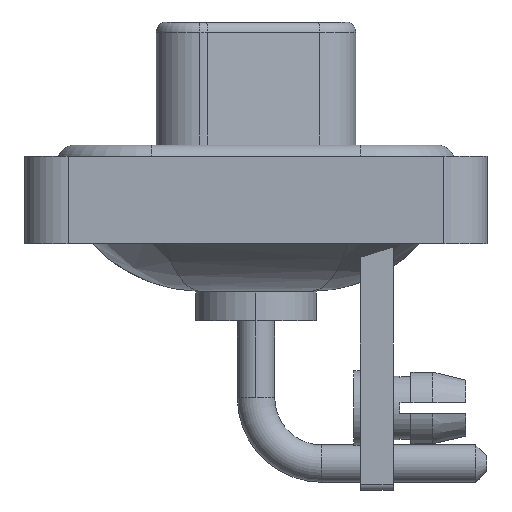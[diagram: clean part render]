
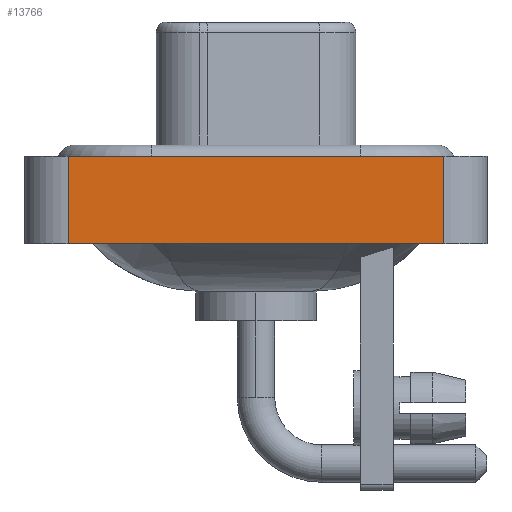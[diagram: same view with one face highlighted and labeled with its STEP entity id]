
A CAD part, left-side view. The second image highlights one B-rep face of the part: STEP entity #13766.
In plain terms, the highlighted planar face has unit normal (-1, 0, 0).
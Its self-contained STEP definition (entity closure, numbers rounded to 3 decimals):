
#1598 = LINE ( 'NONE', #4458, #6937 ) ;
#2211 = VECTOR ( 'NONE', #7094, 1000. ) ;
#2734 = EDGE_CURVE ( 'NONE', #14877, #13758, #1598, .T. ) ;
#2862 = VECTOR ( 'NONE', #9340, 1000. ) ;
#3102 = CARTESIAN_POINT ( 'NONE',  ( -7.25, -8.55, 0.4 ) ) ;
#4458 = CARTESIAN_POINT ( 'NONE',  ( -7.25, -8.55, -3.6 ) ) ;
#4800 = LINE ( 'NONE', #9929, #5241 ) ;
#5241 = VECTOR ( 'NONE', #11504, 1000. ) ;
#5280 = CARTESIAN_POINT ( 'NONE',  ( -7.25, 8.55, -3.6 ) ) ;
#5664 = ORIENTED_EDGE ( 'NONE', *, *, #15489, .F. ) ;
#6180 = CARTESIAN_POINT ( 'NONE',  ( -7.25, -8.55, -3.6 ) ) ;
#6360 = EDGE_CURVE ( 'NONE', #13758, #12039, #4800, .T. ) ;
#6547 = ORIENTED_EDGE ( 'NONE', *, *, #13826, .F. ) ;
#6793 = LINE ( 'NONE', #16657, #2211 ) ;
#6937 = VECTOR ( 'NONE', #7837, 1000. ) ;
#7094 = DIRECTION ( 'NONE',  ( 0., 0., 1. ) ) ;
#7706 = PLANE ( 'NONE',  #18910 ) ;
#7837 = DIRECTION ( 'NONE',  ( 0., -1., 0. ) ) ;
#8452 = CARTESIAN_POINT ( 'NONE',  ( -7.25, 8.55, 0.4 ) ) ;
#9340 = DIRECTION ( 'NONE',  ( 0., -1., 0. ) ) ;
#9929 = CARTESIAN_POINT ( 'NONE',  ( -7.25, -8.55, -3.6 ) ) ;
#11504 = DIRECTION ( 'NONE',  ( 0., 0., 1. ) ) ;
#12039 = VERTEX_POINT ( 'NONE', #12840 ) ;
#12345 = DIRECTION ( 'NONE',  ( 0., 0., 1. ) ) ;
#12840 = CARTESIAN_POINT ( 'NONE',  ( -7.25, -8.55, 0.4 ) ) ;
#13558 = ORIENTED_EDGE ( 'NONE', *, *, #2734, .T. ) ;
#13688 = DIRECTION ( 'NONE',  ( -1., 0., 0. ) ) ;
#13758 = VERTEX_POINT ( 'NONE', #19441 ) ;
#13766 = ADVANCED_FACE ( 'NONE', ( #15431 ), #7706, .T. ) ;
#13826 = EDGE_CURVE ( 'NONE', #16221, #12039, #16968, .T. ) ;
#13921 = ORIENTED_EDGE ( 'NONE', *, *, #6360, .T. ) ;
#14877 = VERTEX_POINT ( 'NONE', #5280 ) ;
#15431 = FACE_OUTER_BOUND ( 'NONE', #17560, .T. ) ;
#15489 = EDGE_CURVE ( 'NONE', #14877, #16221, #6793, .T. ) ;
#16221 = VERTEX_POINT ( 'NONE', #8452 ) ;
#16657 = CARTESIAN_POINT ( 'NONE',  ( -7.25, 8.55, -3.6 ) ) ;
#16968 = LINE ( 'NONE', #3102, #2862 ) ;
#17560 = EDGE_LOOP ( 'NONE', ( #13921, #6547, #5664, #13558 ) ) ;
#18910 = AXIS2_PLACEMENT_3D ( 'NONE', #6180, #13688, #12345 ) ;
#19441 = CARTESIAN_POINT ( 'NONE',  ( -7.25, -8.55, -3.6 ) ) ;
